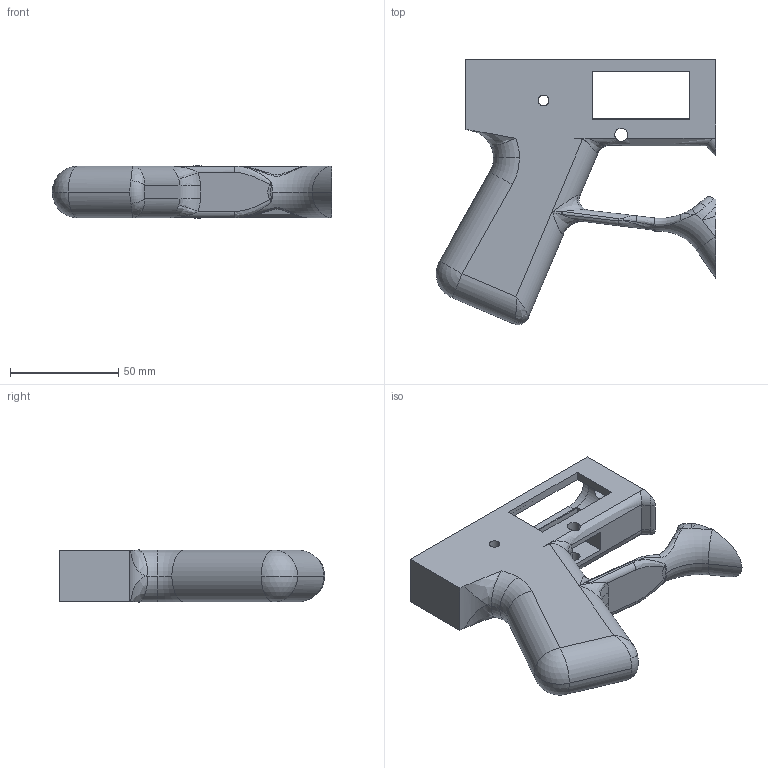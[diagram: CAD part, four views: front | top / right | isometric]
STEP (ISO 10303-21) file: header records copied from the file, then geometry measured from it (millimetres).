
FILE_DESCRIPTION (( 'STEP AP214' ), '1' );
FILE_NAME ('Receiver_Grip_2.step', '2014-05-14T06:10:16', ( 'WarFairy' ), ( '' ), 'SwSTEP 2.0', 'SolidWorks 2013', '' );
FILE_SCHEMA (( 'AUTOMOTIVE_DESIGN' ));
Length unit declared in the file: inch
Products named in the file (1): Receiver_Grip_2
Bounding box: 129.06 x 122.53 x 24.03 mm (x, y, z)
Volume: 159974.8 mm3; surface area: 32642.6 mm2
Topology: 1 solids, 1 shells, 147 faces, 393 edges, 233 vertices
Faces by surface type: bspline 47, cylinder 43, plane 40, torus 11, sphere 6
Entity records: 8452 total; most frequent: CARTESIAN_POINT 5184, ORIENTED_EDGE 762, DIRECTION 572, EDGE_CURVE 381, VERTEX_POINT 233, AXIS2_PLACEMENT_3D 218, EDGE_LOOP 160, ADVANCED_FACE 147
